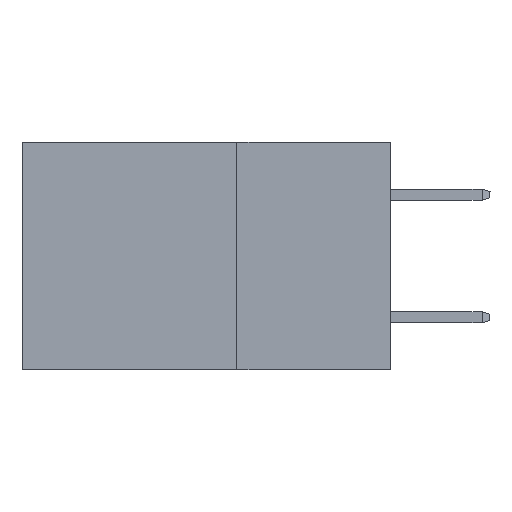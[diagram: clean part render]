
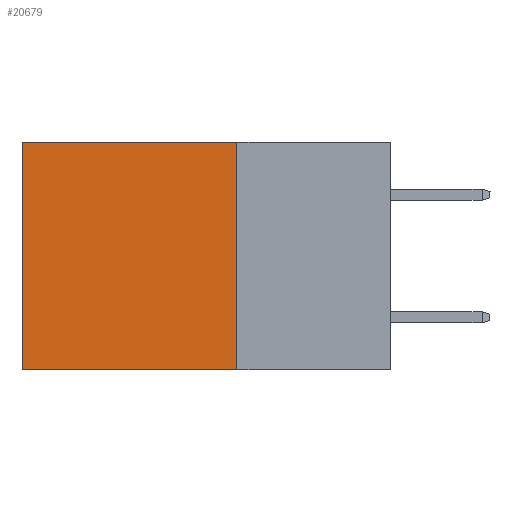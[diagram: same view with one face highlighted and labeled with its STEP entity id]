
A CAD part, left-side view. The second image highlights one B-rep face of the part: STEP entity #20679.
In plain terms, the highlighted planar face has unit normal (-1, 0, 0).
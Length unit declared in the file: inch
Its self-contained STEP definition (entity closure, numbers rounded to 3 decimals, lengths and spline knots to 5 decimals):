
#1016 = CARTESIAN_POINT ( 'NONE',  ( 0.2875, 0.25, -0.37 ) ) ;
#1546 = DIRECTION ( 'NONE',  ( 0., 1., 0. ) ) ;
#3338 = CARTESIAN_POINT ( 'NONE',  ( 0.2875, 0.6, 0. ) ) ;
#6504 = EDGE_CURVE ( 'NONE', #11034, #12943, #10279, .T. ) ;
#7236 = FACE_OUTER_BOUND ( 'NONE', #12457, .T. ) ;
#7559 = VECTOR ( 'NONE', #1546, 39.37008 ) ;
#8512 = ORIENTED_EDGE ( 'NONE', *, *, #15854, .F. ) ;
#9183 = LINE ( 'NONE', #16083, #14713 ) ;
#9290 = DIRECTION ( 'NONE',  ( 0., 0., -1. ) ) ;
#9537 = DIRECTION ( 'NONE',  ( 0., 0., -1. ) ) ;
#9756 = VECTOR ( 'NONE', #14532, 39.37008 ) ;
#10031 = PLANE ( 'NONE',  #13960 ) ;
#10134 = VERTEX_POINT ( 'NONE', #21650 ) ;
#10279 = LINE ( 'NONE', #1016, #9756 ) ;
#10502 = CARTESIAN_POINT ( 'NONE',  ( 0.2875, 0.6, -0.37 ) ) ;
#11034 = VERTEX_POINT ( 'NONE', #17345 ) ;
#12070 = DIRECTION ( 'NONE',  ( 1., 0., 0. ) ) ;
#12385 = ORIENTED_EDGE ( 'NONE', *, *, #14420, .T. ) ;
#12456 = DIRECTION ( 'NONE',  ( 0., 0., -1. ) ) ;
#12457 = EDGE_LOOP ( 'NONE', ( #17922, #21351, #8512, #12385 ) ) ;
#12508 = VECTOR ( 'NONE', #12456, 39.37008 ) ;
#12943 = VERTEX_POINT ( 'NONE', #10502 ) ;
#13536 = EDGE_CURVE ( 'NONE', #20100, #12943, #9183, .T. ) ;
#13902 = CARTESIAN_POINT ( 'NONE',  ( 0.2875, 0.25, 0. ) ) ;
#13960 = AXIS2_PLACEMENT_3D ( 'NONE', #13902, #12070, #9537 ) ;
#14273 = CARTESIAN_POINT ( 'NONE',  ( 0.2875, 0.25, 0. ) ) ;
#14420 = EDGE_CURVE ( 'NONE', #10134, #20100, #16000, .T. ) ;
#14532 = DIRECTION ( 'NONE',  ( 0., 1., 0. ) ) ;
#14713 = VECTOR ( 'NONE', #9290, 39.37008 ) ;
#15854 = EDGE_CURVE ( 'NONE', #10134, #11034, #16194, .T. ) ;
#16000 = LINE ( 'NONE', #21782, #7559 ) ;
#16083 = CARTESIAN_POINT ( 'NONE',  ( 0.2875, 0.6, 0. ) ) ;
#16194 = LINE ( 'NONE', #14273, #12508 ) ;
#17345 = CARTESIAN_POINT ( 'NONE',  ( 0.2875, 0.25, -0.37 ) ) ;
#17922 = ORIENTED_EDGE ( 'NONE', *, *, #13536, .T. ) ;
#20100 = VERTEX_POINT ( 'NONE', #3338 ) ;
#20679 = ADVANCED_FACE ( 'NONE', ( #7236 ), #10031, .F. ) ;
#21351 = ORIENTED_EDGE ( 'NONE', *, *, #6504, .F. ) ;
#21650 = CARTESIAN_POINT ( 'NONE',  ( 0.2875, 0.25, 0. ) ) ;
#21782 = CARTESIAN_POINT ( 'NONE',  ( 0.2875, 0.25, 0. ) ) ;
